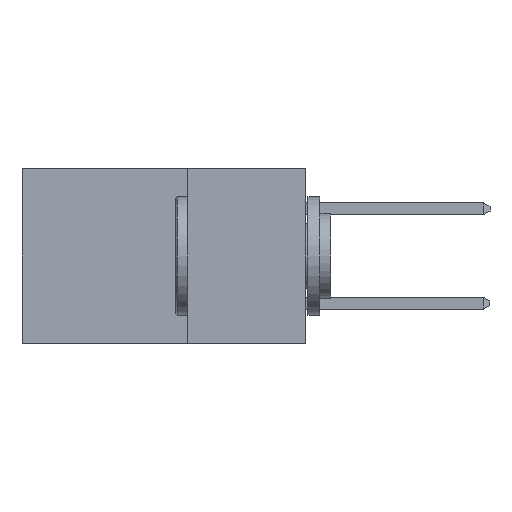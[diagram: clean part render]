
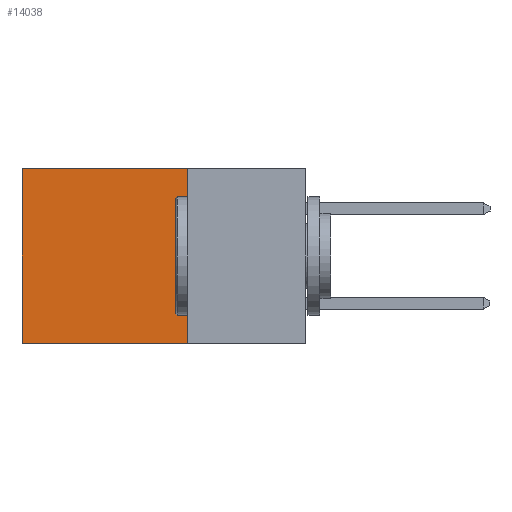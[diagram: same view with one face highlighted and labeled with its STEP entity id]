
A CAD part, left-side view. The second image highlights one B-rep face of the part: STEP entity #14038.
In plain terms, the highlighted planar face has unit normal (-1, 0, 0).
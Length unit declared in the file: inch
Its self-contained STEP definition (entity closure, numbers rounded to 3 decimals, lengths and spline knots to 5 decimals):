
#117 = EDGE_CURVE ( 'NONE', #13414, #12849, #11524, .T. ) ;
#231 = CARTESIAN_POINT ( 'NONE',  ( 0.298, 0.25, 0. ) ) ;
#1104 = AXIS2_PLACEMENT_3D ( 'NONE', #231, #9220, #1496 ) ;
#1496 = DIRECTION ( 'NONE',  ( 0., 0., -1. ) ) ;
#2577 = CARTESIAN_POINT ( 'NONE',  ( 0.298, 0.25, 0. ) ) ;
#3552 = VERTEX_POINT ( 'NONE', #15432 ) ;
#3699 = VECTOR ( 'NONE', #7541, 39.37008 ) ;
#3822 = DIRECTION ( 'NONE',  ( 0., 1., 0. ) ) ;
#4127 = LINE ( 'NONE', #6273, #3699 ) ;
#5150 = CARTESIAN_POINT ( 'NONE',  ( 0.298, 0.25, -0.37 ) ) ;
#5587 = VECTOR ( 'NONE', #3822, 39.37008 ) ;
#6273 = CARTESIAN_POINT ( 'NONE',  ( 0.298, 0.25, 0. ) ) ;
#6999 = ORIENTED_EDGE ( 'NONE', *, *, #117, .F. ) ;
#7273 = EDGE_LOOP ( 'NONE', ( #11468, #9064, #6999, #9238 ) ) ;
#7541 = DIRECTION ( 'NONE',  ( 0., 1., 0. ) ) ;
#7942 = CARTESIAN_POINT ( 'NONE',  ( 0.298, 0.25, -0.37 ) ) ;
#7963 = PLANE ( 'NONE',  #1104 ) ;
#8317 = VECTOR ( 'NONE', #9983, 39.37008 ) ;
#8713 = LINE ( 'NONE', #8720, #8317 ) ;
#8720 = CARTESIAN_POINT ( 'NONE',  ( 0.298, 0.6, 0. ) ) ;
#9064 = ORIENTED_EDGE ( 'NONE', *, *, #9271, .F. ) ;
#9220 = DIRECTION ( 'NONE',  ( 1., 0., 0. ) ) ;
#9238 = ORIENTED_EDGE ( 'NONE', *, *, #10471, .T. ) ;
#9271 = EDGE_CURVE ( 'NONE', #12849, #11154, #15627, .T. ) ;
#9983 = DIRECTION ( 'NONE',  ( 0., 0., -1. ) ) ;
#10471 = EDGE_CURVE ( 'NONE', #13414, #3552, #4127, .T. ) ;
#10523 = DIRECTION ( 'NONE',  ( 0., 0., -1. ) ) ;
#11154 = VERTEX_POINT ( 'NONE', #13713 ) ;
#11468 = ORIENTED_EDGE ( 'NONE', *, *, #11896, .T. ) ;
#11524 = LINE ( 'NONE', #16161, #14490 ) ;
#11896 = EDGE_CURVE ( 'NONE', #3552, #11154, #8713, .T. ) ;
#12849 = VERTEX_POINT ( 'NONE', #7942 ) ;
#13414 = VERTEX_POINT ( 'NONE', #2577 ) ;
#13713 = CARTESIAN_POINT ( 'NONE',  ( 0.298, 0.6, -0.37 ) ) ;
#14038 = ADVANCED_FACE ( 'NONE', ( #16101 ), #7963, .F. ) ;
#14490 = VECTOR ( 'NONE', #10523, 39.37008 ) ;
#15432 = CARTESIAN_POINT ( 'NONE',  ( 0.298, 0.6, 0. ) ) ;
#15627 = LINE ( 'NONE', #5150, #5587 ) ;
#16101 = FACE_OUTER_BOUND ( 'NONE', #7273, .T. ) ;
#16161 = CARTESIAN_POINT ( 'NONE',  ( 0.298, 0.25, 0. ) ) ;
